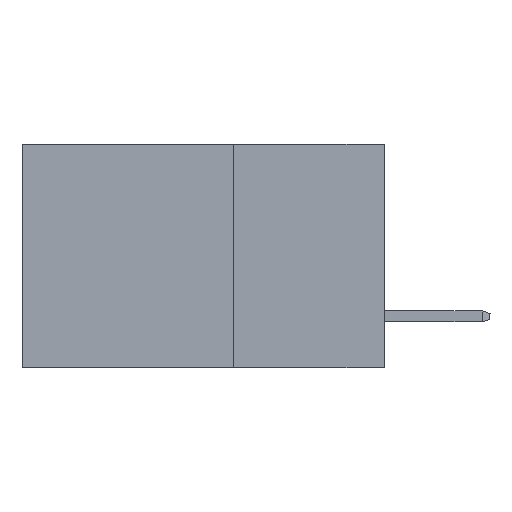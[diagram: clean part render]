
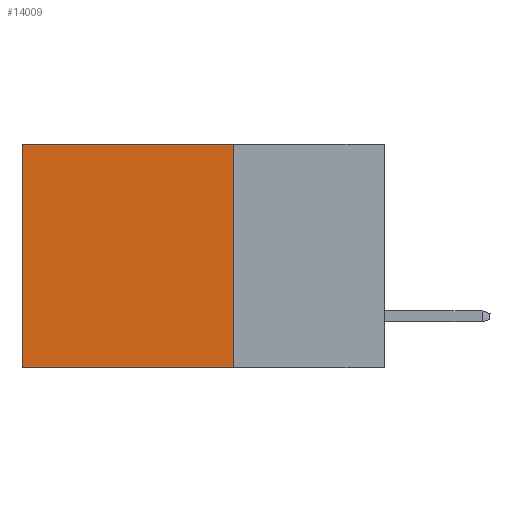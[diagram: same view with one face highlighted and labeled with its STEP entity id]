
A CAD part, left-side view. The second image highlights one B-rep face of the part: STEP entity #14009.
In plain terms, the highlighted planar face has unit normal (-1, 0, 0).
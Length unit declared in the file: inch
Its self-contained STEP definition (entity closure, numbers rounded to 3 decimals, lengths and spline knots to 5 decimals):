
#80 = EDGE_LOOP ( 'NONE', ( #15483, #17891, #18212, #10421 ) ) ;
#1204 = VERTEX_POINT ( 'NONE', #3900 ) ;
#1743 = CARTESIAN_POINT ( 'NONE',  ( 0.2615, 0.25, -0.37 ) ) ;
#2022 = CARTESIAN_POINT ( 'NONE',  ( 0.2615, 0.25, 0. ) ) ;
#2371 = LINE ( 'NONE', #19353, #10390 ) ;
#3269 = VERTEX_POINT ( 'NONE', #2022 ) ;
#3900 = CARTESIAN_POINT ( 'NONE',  ( 0.2615, 0.6, -0.37 ) ) ;
#4795 = LINE ( 'NONE', #17140, #19631 ) ;
#5657 = EDGE_CURVE ( 'NONE', #3269, #7499, #18304, .T. ) ;
#6629 = DIRECTION ( 'NONE',  ( 0., 0., -1. ) ) ;
#7499 = VERTEX_POINT ( 'NONE', #7890 ) ;
#7525 = LINE ( 'NONE', #9155, #18910 ) ;
#7890 = CARTESIAN_POINT ( 'NONE',  ( 0.2615, 0.6, 0. ) ) ;
#8687 = EDGE_CURVE ( 'NONE', #7499, #1204, #2371, .T. ) ;
#9155 = CARTESIAN_POINT ( 'NONE',  ( 0.2615, 0.25, -0.37 ) ) ;
#9179 = DIRECTION ( 'NONE',  ( 0., 0., -1. ) ) ;
#9449 = VERTEX_POINT ( 'NONE', #1743 ) ;
#9978 = FACE_OUTER_BOUND ( 'NONE', #80, .T. ) ;
#10263 = CARTESIAN_POINT ( 'NONE',  ( 0.2615, 0.25, 0. ) ) ;
#10390 = VECTOR ( 'NONE', #11685, 39.37008 ) ;
#10421 = ORIENTED_EDGE ( 'NONE', *, *, #5657, .T. ) ;
#11140 = AXIS2_PLACEMENT_3D ( 'NONE', #18861, #15727, #6629 ) ;
#11276 = VECTOR ( 'NONE', #16308, 39.37008 ) ;
#11685 = DIRECTION ( 'NONE',  ( 0., 0., -1. ) ) ;
#13704 = DIRECTION ( 'NONE',  ( 0., 1., 0. ) ) ;
#14009 = ADVANCED_FACE ( 'NONE', ( #9978 ), #17241, .F. ) ;
#15483 = ORIENTED_EDGE ( 'NONE', *, *, #8687, .T. ) ;
#15608 = EDGE_CURVE ( 'NONE', #9449, #1204, #7525, .T. ) ;
#15727 = DIRECTION ( 'NONE',  ( 1., 0., 0. ) ) ;
#16308 = DIRECTION ( 'NONE',  ( 0., 1., 0. ) ) ;
#17140 = CARTESIAN_POINT ( 'NONE',  ( 0.2615, 0.25, -0.37 ) ) ;
#17241 = PLANE ( 'NONE',  #11140 ) ;
#17891 = ORIENTED_EDGE ( 'NONE', *, *, #15608, .F. ) ;
#18212 = ORIENTED_EDGE ( 'NONE', *, *, #19584, .F. ) ;
#18304 = LINE ( 'NONE', #10263, #11276 ) ;
#18861 = CARTESIAN_POINT ( 'NONE',  ( 0.2615, 0.25, -0.37 ) ) ;
#18910 = VECTOR ( 'NONE', #13704, 39.37008 ) ;
#19353 = CARTESIAN_POINT ( 'NONE',  ( 0.2615, 0.6, -0.37 ) ) ;
#19584 = EDGE_CURVE ( 'NONE', #3269, #9449, #4795, .T. ) ;
#19631 = VECTOR ( 'NONE', #9179, 39.37008 ) ;
